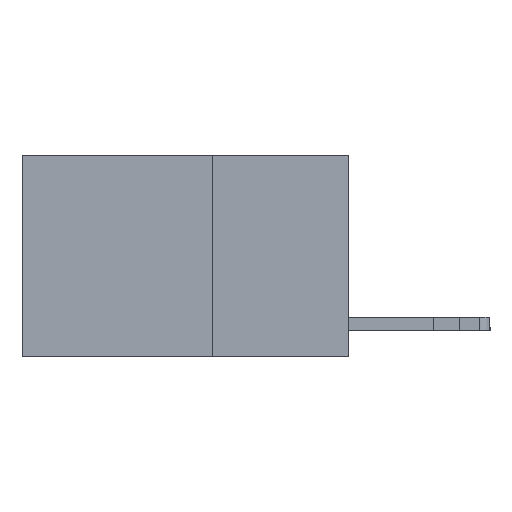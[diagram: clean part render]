
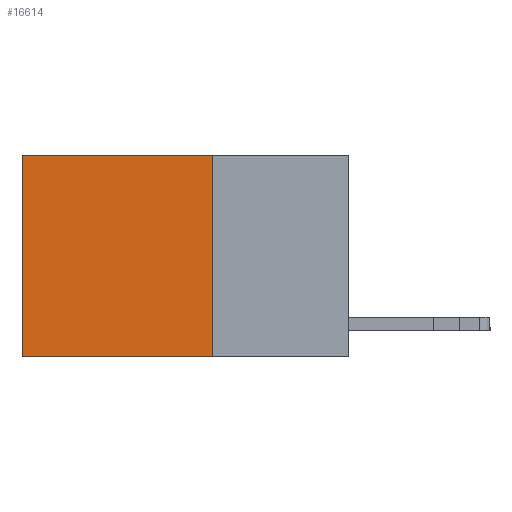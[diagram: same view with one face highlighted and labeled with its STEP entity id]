
A CAD part, left-side view. The second image highlights one B-rep face of the part: STEP entity #16614.
In plain terms, the highlighted planar face has unit normal (-1, 0, 0).
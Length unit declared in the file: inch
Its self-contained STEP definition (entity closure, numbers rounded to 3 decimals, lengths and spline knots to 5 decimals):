
#128 = AXIS2_PLACEMENT_3D ( 'NONE', #21139, #19937, #16719 ) ;
#412 = CARTESIAN_POINT ( 'NONE',  ( 0.2625, 0.6, 0. ) ) ;
#1353 = FACE_OUTER_BOUND ( 'NONE', #17624, .T. ) ;
#1392 = EDGE_CURVE ( 'NONE', #3149, #7261, #12280, .T. ) ;
#1916 = CARTESIAN_POINT ( 'NONE',  ( 0.2625, 0.25, -0.37 ) ) ;
#2793 = EDGE_CURVE ( 'NONE', #3149, #10959, #15369, .T. ) ;
#3149 = VERTEX_POINT ( 'NONE', #5580 ) ;
#4864 = VECTOR ( 'NONE', #8397, 39.37008 ) ;
#5580 = CARTESIAN_POINT ( 'NONE',  ( 0.2625, 0.25, 0. ) ) ;
#6325 = VECTOR ( 'NONE', #16955, 39.37008 ) ;
#7261 = VERTEX_POINT ( 'NONE', #9937 ) ;
#7918 = PLANE ( 'NONE',  #128 ) ;
#8397 = DIRECTION ( 'NONE',  ( 0., 0., -1. ) ) ;
#9755 = CARTESIAN_POINT ( 'NONE',  ( 0.2625, 0.6, -0.37 ) ) ;
#9903 = ORIENTED_EDGE ( 'NONE', *, *, #20958, .T. ) ;
#9937 = CARTESIAN_POINT ( 'NONE',  ( 0.2625, 0.25, -0.37 ) ) ;
#10144 = VERTEX_POINT ( 'NONE', #9755 ) ;
#10583 = CARTESIAN_POINT ( 'NONE',  ( 0.2625, 0.25, 0. ) ) ;
#10959 = VERTEX_POINT ( 'NONE', #12640 ) ;
#12280 = LINE ( 'NONE', #18686, #21041 ) ;
#12640 = CARTESIAN_POINT ( 'NONE',  ( 0.2625, 0.6, 0. ) ) ;
#13903 = ORIENTED_EDGE ( 'NONE', *, *, #16292, .F. ) ;
#14998 = LINE ( 'NONE', #1916, #6325 ) ;
#15369 = LINE ( 'NONE', #10583, #20195 ) ;
#16292 = EDGE_CURVE ( 'NONE', #7261, #10144, #14998, .T. ) ;
#16614 = ADVANCED_FACE ( 'NONE', ( #1353 ), #7918, .F. ) ;
#16719 = DIRECTION ( 'NONE',  ( 0., 0., -1. ) ) ;
#16887 = DIRECTION ( 'NONE',  ( 0., 1., 0. ) ) ;
#16955 = DIRECTION ( 'NONE',  ( 0., 1., 0. ) ) ;
#17339 = ORIENTED_EDGE ( 'NONE', *, *, #2793, .T. ) ;
#17624 = EDGE_LOOP ( 'NONE', ( #9903, #13903, #20008, #17339 ) ) ;
#18686 = CARTESIAN_POINT ( 'NONE',  ( 0.2625, 0.25, 0. ) ) ;
#18901 = DIRECTION ( 'NONE',  ( 0., 0., -1. ) ) ;
#19877 = LINE ( 'NONE', #412, #4864 ) ;
#19937 = DIRECTION ( 'NONE',  ( 1., 0., 0. ) ) ;
#20008 = ORIENTED_EDGE ( 'NONE', *, *, #1392, .F. ) ;
#20195 = VECTOR ( 'NONE', #16887, 39.37008 ) ;
#20958 = EDGE_CURVE ( 'NONE', #10959, #10144, #19877, .T. ) ;
#21041 = VECTOR ( 'NONE', #18901, 39.37008 ) ;
#21139 = CARTESIAN_POINT ( 'NONE',  ( 0.2625, 0.25, 0. ) ) ;
